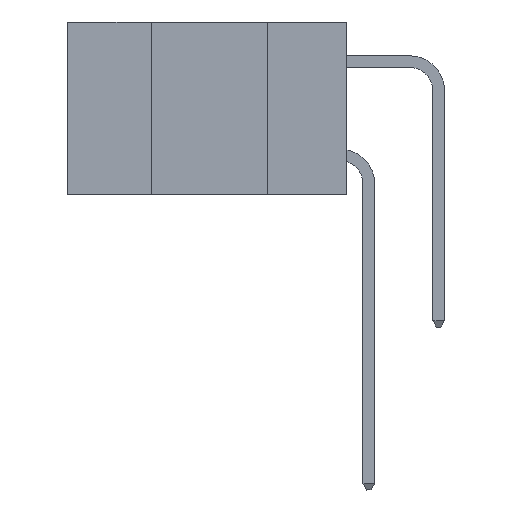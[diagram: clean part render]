
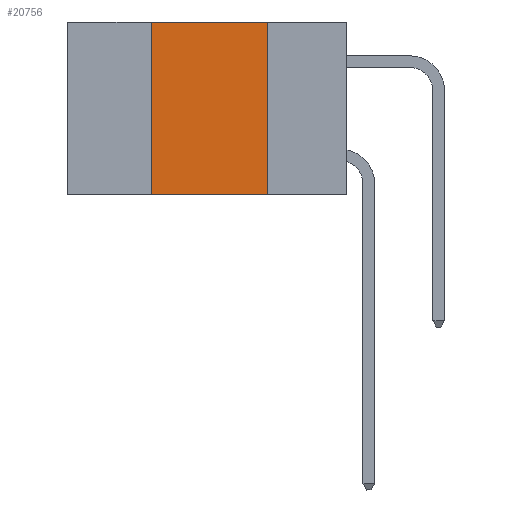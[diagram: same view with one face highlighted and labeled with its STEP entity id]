
A CAD part, left-side view. The second image highlights one B-rep face of the part: STEP entity #20756.
In plain terms, the highlighted planar face has unit normal (-1, 0, 0).
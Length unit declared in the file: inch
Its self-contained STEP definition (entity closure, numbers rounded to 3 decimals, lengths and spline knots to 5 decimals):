
#767 = ORIENTED_EDGE ( 'NONE', *, *, #921, .F. ) ;
#921 = EDGE_CURVE ( 'NONE', #13624, #15895, #26520, .T. ) ;
#2791 = VERTEX_POINT ( 'NONE', #33954 ) ;
#3012 = LINE ( 'NONE', #6822, #13689 ) ;
#3249 = CARTESIAN_POINT ( 'NONE',  ( 0., 0.17, 0. ) ) ;
#3385 = VERTEX_POINT ( 'NONE', #17306 ) ;
#3657 = ORIENTED_EDGE ( 'NONE', *, *, #24868, .F. ) ;
#3682 = PLANE ( 'NONE',  #10130 ) ;
#3911 = VECTOR ( 'NONE', #25436, 39.37008 ) ;
#6405 = CARTESIAN_POINT ( 'NONE',  ( 0., 0.17, 0. ) ) ;
#6822 = CARTESIAN_POINT ( 'NONE',  ( 0., 0.42, 0. ) ) ;
#6926 = CARTESIAN_POINT ( 'NONE',  ( 0., 0.6, 0. ) ) ;
#10051 = LINE ( 'NONE', #3249, #30663 ) ;
#10130 = AXIS2_PLACEMENT_3D ( 'NONE', #32951, #16873, #25186 ) ;
#12546 = DIRECTION ( 'NONE',  ( 0., -1., 0. ) ) ;
#13220 = VECTOR ( 'NONE', #12546, 39.37008 ) ;
#13624 = VERTEX_POINT ( 'NONE', #28002 ) ;
#13689 = VECTOR ( 'NONE', #30535, 39.37008 ) ;
#15895 = VERTEX_POINT ( 'NONE', #6405 ) ;
#16873 = DIRECTION ( 'NONE',  ( 1., 0., 0. ) ) ;
#17306 = CARTESIAN_POINT ( 'NONE',  ( 0., 0.42, -0.37 ) ) ;
#17336 = LINE ( 'NONE', #28102, #13220 ) ;
#19555 = EDGE_LOOP ( 'NONE', ( #3657, #767, #26840, #24789 ) ) ;
#20756 = ADVANCED_FACE ( 'NONE', ( #29086 ), #3682, .F. ) ;
#24789 = ORIENTED_EDGE ( 'NONE', *, *, #32280, .T. ) ;
#24868 = EDGE_CURVE ( 'NONE', #15895, #2791, #10051, .T. ) ;
#25186 = DIRECTION ( 'NONE',  ( 0., 0., -1. ) ) ;
#25198 = EDGE_CURVE ( 'NONE', #3385, #13624, #3012, .T. ) ;
#25436 = DIRECTION ( 'NONE',  ( 0., -1., 0. ) ) ;
#26520 = LINE ( 'NONE', #6926, #3911 ) ;
#26840 = ORIENTED_EDGE ( 'NONE', *, *, #25198, .F. ) ;
#28002 = CARTESIAN_POINT ( 'NONE',  ( 0., 0.42, 0. ) ) ;
#28102 = CARTESIAN_POINT ( 'NONE',  ( 0., 0.6, -0.37 ) ) ;
#29086 = FACE_OUTER_BOUND ( 'NONE', #19555, .T. ) ;
#30535 = DIRECTION ( 'NONE',  ( 0., 0., 1. ) ) ;
#30663 = VECTOR ( 'NONE', #31816, 39.37008 ) ;
#31816 = DIRECTION ( 'NONE',  ( 0., 0., -1. ) ) ;
#32280 = EDGE_CURVE ( 'NONE', #3385, #2791, #17336, .T. ) ;
#32951 = CARTESIAN_POINT ( 'NONE',  ( 0., 0.6, 0. ) ) ;
#33954 = CARTESIAN_POINT ( 'NONE',  ( 0., 0.17, -0.37 ) ) ;
